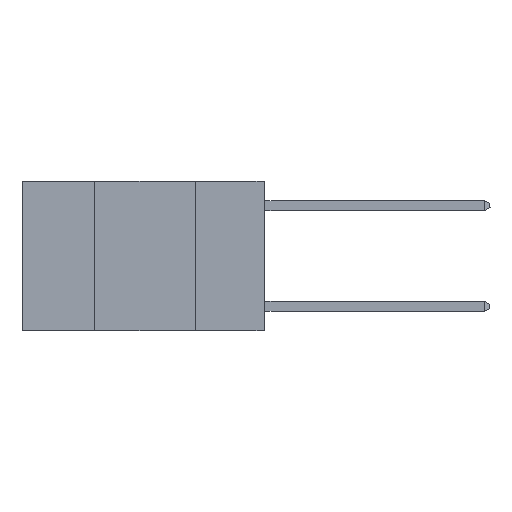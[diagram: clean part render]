
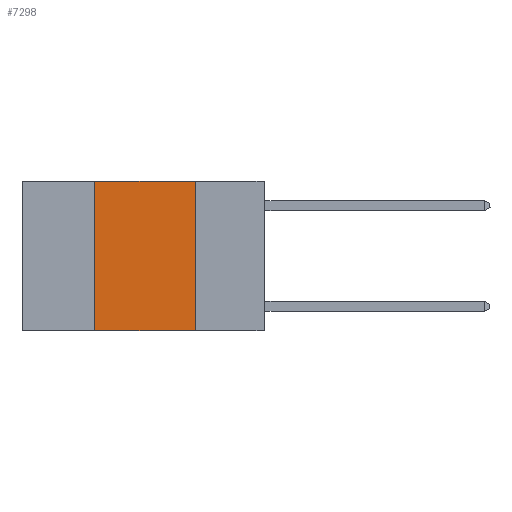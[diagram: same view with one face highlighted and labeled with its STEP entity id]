
A CAD part, left-side view. The second image highlights one B-rep face of the part: STEP entity #7298.
In plain terms, the highlighted planar face has unit normal (-1, 0, 0).
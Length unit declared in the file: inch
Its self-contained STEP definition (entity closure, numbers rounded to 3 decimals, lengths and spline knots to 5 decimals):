
#133 = CARTESIAN_POINT ( 'NONE',  ( 0., 0.6, 0. ) ) ;
#1290 = AXIS2_PLACEMENT_3D ( 'NONE', #133, #2052, #14990 ) ;
#1731 = LINE ( 'NONE', #14422, #20848 ) ;
#1952 = VERTEX_POINT ( 'NONE', #12809 ) ;
#2017 = CARTESIAN_POINT ( 'NONE',  ( 0., 0.17, -0.37 ) ) ;
#2052 = DIRECTION ( 'NONE',  ( 1., 0., 0. ) ) ;
#2300 = ORIENTED_EDGE ( 'NONE', *, *, #22690, .F. ) ;
#7298 = ADVANCED_FACE ( 'NONE', ( #21556 ), #11258, .F. ) ;
#7526 = LINE ( 'NONE', #14531, #21691 ) ;
#8005 = LINE ( 'NONE', #17702, #17227 ) ;
#8421 = CARTESIAN_POINT ( 'NONE',  ( 0., 0.42, 0. ) ) ;
#8526 = DIRECTION ( 'NONE',  ( 0., 0., -1. ) ) ;
#10981 = EDGE_CURVE ( 'NONE', #1952, #23505, #8005, .T. ) ;
#11258 = PLANE ( 'NONE',  #1290 ) ;
#12108 = ORIENTED_EDGE ( 'NONE', *, *, #15596, .F. ) ;
#12616 = DIRECTION ( 'NONE',  ( 0., -1., 0. ) ) ;
#12809 = CARTESIAN_POINT ( 'NONE',  ( 0., 0.17, 0. ) ) ;
#13935 = EDGE_CURVE ( 'NONE', #15543, #23505, #18850, .T. ) ;
#14422 = CARTESIAN_POINT ( 'NONE',  ( 0., 0.6, 0. ) ) ;
#14531 = CARTESIAN_POINT ( 'NONE',  ( 0., 0.42, 0. ) ) ;
#14990 = DIRECTION ( 'NONE',  ( 0., 0., -1. ) ) ;
#15328 = CARTESIAN_POINT ( 'NONE',  ( 0., 0.6, -0.37 ) ) ;
#15543 = VERTEX_POINT ( 'NONE', #18047 ) ;
#15596 = EDGE_CURVE ( 'NONE', #15543, #23142, #7526, .T. ) ;
#15879 = ORIENTED_EDGE ( 'NONE', *, *, #10981, .F. ) ;
#17151 = DIRECTION ( 'NONE',  ( 0., -1., 0. ) ) ;
#17227 = VECTOR ( 'NONE', #8526, 39.37008 ) ;
#17702 = CARTESIAN_POINT ( 'NONE',  ( 0., 0.17, 0. ) ) ;
#18047 = CARTESIAN_POINT ( 'NONE',  ( 0., 0.42, -0.37 ) ) ;
#18210 = DIRECTION ( 'NONE',  ( 0., 0., 1. ) ) ;
#18850 = LINE ( 'NONE', #15328, #23175 ) ;
#20848 = VECTOR ( 'NONE', #12616, 39.37008 ) ;
#21556 = FACE_OUTER_BOUND ( 'NONE', #23461, .T. ) ;
#21691 = VECTOR ( 'NONE', #18210, 39.37008 ) ;
#21967 = ORIENTED_EDGE ( 'NONE', *, *, #13935, .T. ) ;
#22690 = EDGE_CURVE ( 'NONE', #23142, #1952, #1731, .T. ) ;
#23142 = VERTEX_POINT ( 'NONE', #8421 ) ;
#23175 = VECTOR ( 'NONE', #17151, 39.37008 ) ;
#23461 = EDGE_LOOP ( 'NONE', ( #15879, #2300, #12108, #21967 ) ) ;
#23505 = VERTEX_POINT ( 'NONE', #2017 ) ;
